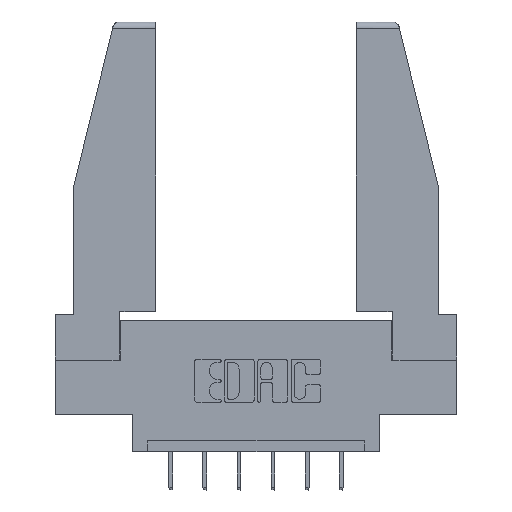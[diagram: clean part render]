
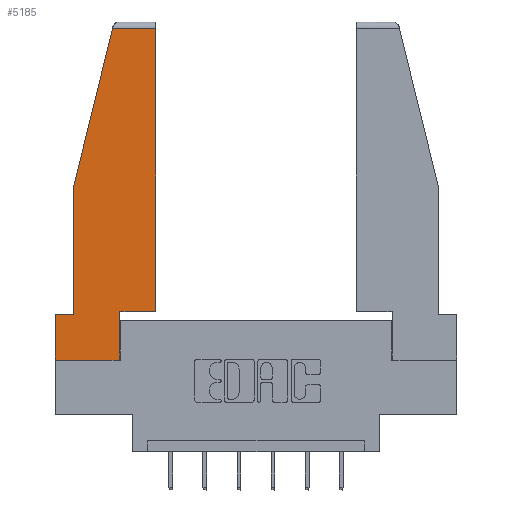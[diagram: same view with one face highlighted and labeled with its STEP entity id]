
A CAD part, top view. The second image highlights one B-rep face of the part: STEP entity #5185.
In plain terms, the highlighted planar face has unit normal (0, 0, 1).
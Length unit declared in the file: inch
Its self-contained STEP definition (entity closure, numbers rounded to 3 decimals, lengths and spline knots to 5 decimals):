
#252 = CARTESIAN_POINT ( 'NONE',  ( 0.297, 0.223, 0. ) ) ;
#356 = DIRECTION ( 'NONE',  ( -1., 0., 0. ) ) ;
#524 = EDGE_CURVE ( 'NONE', #5248, #5823, #3698, .T. ) ;
#767 = CARTESIAN_POINT ( 'NONE',  ( 0.461, 1.52, 0. ) ) ;
#806 = EDGE_CURVE ( 'NONE', #8979, #3848, #6257, .T. ) ;
#948 = CARTESIAN_POINT ( 'NONE',  ( 0.297, 0., 0. ) ) ;
#1561 = CARTESIAN_POINT ( 'NONE',  ( 0., 0., 0. ) ) ;
#1620 = DIRECTION ( 'NONE',  ( 0., -1., 0. ) ) ;
#1641 = ORIENTED_EDGE ( 'NONE', *, *, #2174, .T. ) ;
#1899 = ORIENTED_EDGE ( 'NONE', *, *, #524, .T. ) ;
#1971 = ORIENTED_EDGE ( 'NONE', *, *, #10494, .T. ) ;
#2000 = DIRECTION ( 'NONE',  ( 1., 0., 0. ) ) ;
#2039 = AXIS2_PLACEMENT_3D ( 'NONE', #8270, #2852, #2000 ) ;
#2093 = CARTESIAN_POINT ( 'NONE',  ( 0., 0.21, 0. ) ) ;
#2174 = EDGE_CURVE ( 'NONE', #9119, #4191, #6309, .T. ) ;
#2256 = EDGE_CURVE ( 'NONE', #3305, #8914, #4735, .T. ) ;
#2613 = CARTESIAN_POINT ( 'NONE',  ( 0., 0.21, 0. ) ) ;
#2693 = VECTOR ( 'NONE', #8449, 39.37008 ) ;
#2811 = PLANE ( 'NONE',  #2039 ) ;
#2823 = DIRECTION ( 'NONE',  ( 0., 1., 0. ) ) ;
#2852 = DIRECTION ( 'NONE',  ( 0., 0., 1. ) ) ;
#3189 = VECTOR ( 'NONE', #11757, 39.37008 ) ;
#3195 = LINE ( 'NONE', #948, #3353 ) ;
#3305 = VERTEX_POINT ( 'NONE', #10731 ) ;
#3353 = VECTOR ( 'NONE', #2823, 39.37008 ) ;
#3360 = CARTESIAN_POINT ( 'NONE',  ( 0., 0., 0. ) ) ;
#3698 = LINE ( 'NONE', #3360, #6677 ) ;
#3848 = VERTEX_POINT ( 'NONE', #7847 ) ;
#3872 = ORIENTED_EDGE ( 'NONE', *, *, #806, .T. ) ;
#4191 = VERTEX_POINT ( 'NONE', #4958 ) ;
#4601 = EDGE_CURVE ( 'NONE', #8914, #5248, #9980, .T. ) ;
#4628 = DIRECTION ( 'NONE',  ( 0., 1., 0. ) ) ;
#4735 = LINE ( 'NONE', #5455, #8179 ) ;
#4824 = DIRECTION ( 'NONE',  ( -0.239, -0.971, 0. ) ) ;
#4958 = CARTESIAN_POINT ( 'NONE',  ( 0.461, 0.223, 0. ) ) ;
#5185 = ADVANCED_FACE ( 'NONE', ( #7962 ), #2811, .T. ) ;
#5248 = VERTEX_POINT ( 'NONE', #1561 ) ;
#5455 = CARTESIAN_POINT ( 'NONE',  ( 0., 0.21, 0. ) ) ;
#5720 = VECTOR ( 'NONE', #1620, 39.37008 ) ;
#5823 = VERTEX_POINT ( 'NONE', #10764 ) ;
#5978 = VECTOR ( 'NONE', #4628, 39.37008 ) ;
#6257 = LINE ( 'NONE', #7677, #10117 ) ;
#6309 = LINE ( 'NONE', #9746, #3189 ) ;
#6373 = DIRECTION ( 'NONE',  ( -1., 0., 0. ) ) ;
#6417 = LINE ( 'NONE', #6969, #5978 ) ;
#6447 = LINE ( 'NONE', #10383, #9589 ) ;
#6677 = VECTOR ( 'NONE', #10725, 39.37008 ) ;
#6969 = CARTESIAN_POINT ( 'NONE',  ( 0.461, 0.223, 0. ) ) ;
#7030 = ORIENTED_EDGE ( 'NONE', *, *, #9960, .T. ) ;
#7267 = ORIENTED_EDGE ( 'NONE', *, *, #9120, .T. ) ;
#7306 = ORIENTED_EDGE ( 'NONE', *, *, #2256, .T. ) ;
#7677 = CARTESIAN_POINT ( 'NONE',  ( 0., 1.52, 0. ) ) ;
#7847 = CARTESIAN_POINT ( 'NONE',  ( 0.2636, 1.52, 0. ) ) ;
#7962 = FACE_OUTER_BOUND ( 'NONE', #8321, .T. ) ;
#8167 = EDGE_CURVE ( 'NONE', #5823, #9119, #3195, .T. ) ;
#8179 = VECTOR ( 'NONE', #6373, 39.37008 ) ;
#8270 = CARTESIAN_POINT ( 'NONE',  ( 0., 0., 0. ) ) ;
#8321 = EDGE_LOOP ( 'NONE', ( #1971, #3872, #7267, #7030, #7306, #11327, #1899, #10209, #1641 ) ) ;
#8449 = DIRECTION ( 'NONE',  ( 0., -1., 0. ) ) ;
#8582 = LINE ( 'NONE', #10547, #5720 ) ;
#8914 = VERTEX_POINT ( 'NONE', #2613 ) ;
#8979 = VERTEX_POINT ( 'NONE', #767 ) ;
#9119 = VERTEX_POINT ( 'NONE', #252 ) ;
#9120 = EDGE_CURVE ( 'NONE', #3848, #11481, #6447, .T. ) ;
#9589 = VECTOR ( 'NONE', #4824, 39.37008 ) ;
#9590 = CARTESIAN_POINT ( 'NONE',  ( 0.086, 0.8, 0. ) ) ;
#9746 = CARTESIAN_POINT ( 'NONE',  ( 0.297, 0.223, 0. ) ) ;
#9960 = EDGE_CURVE ( 'NONE', #11481, #3305, #8582, .T. ) ;
#9980 = LINE ( 'NONE', #2093, #2693 ) ;
#10117 = VECTOR ( 'NONE', #356, 39.37008 ) ;
#10209 = ORIENTED_EDGE ( 'NONE', *, *, #8167, .T. ) ;
#10383 = CARTESIAN_POINT ( 'NONE',  ( 0.271, 1.55, 0. ) ) ;
#10494 = EDGE_CURVE ( 'NONE', #4191, #8979, #6417, .T. ) ;
#10547 = CARTESIAN_POINT ( 'NONE',  ( 0.086, 0.8, 0. ) ) ;
#10725 = DIRECTION ( 'NONE',  ( 1., 0., 0. ) ) ;
#10731 = CARTESIAN_POINT ( 'NONE',  ( 0.086, 0.21, 0. ) ) ;
#10764 = CARTESIAN_POINT ( 'NONE',  ( 0.297, 0., 0. ) ) ;
#11327 = ORIENTED_EDGE ( 'NONE', *, *, #4601, .T. ) ;
#11481 = VERTEX_POINT ( 'NONE', #9590 ) ;
#11757 = DIRECTION ( 'NONE',  ( 1., 0., 0. ) ) ;
